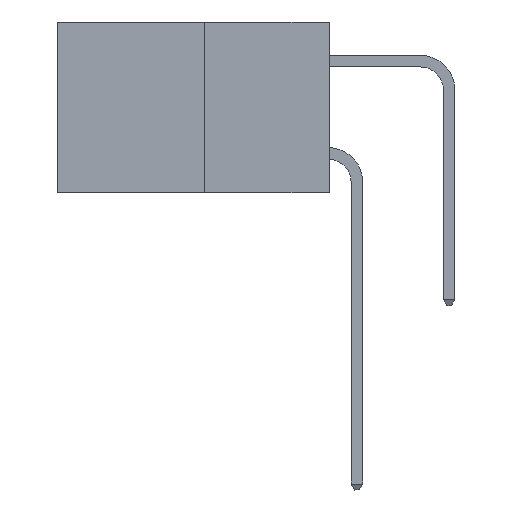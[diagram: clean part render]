
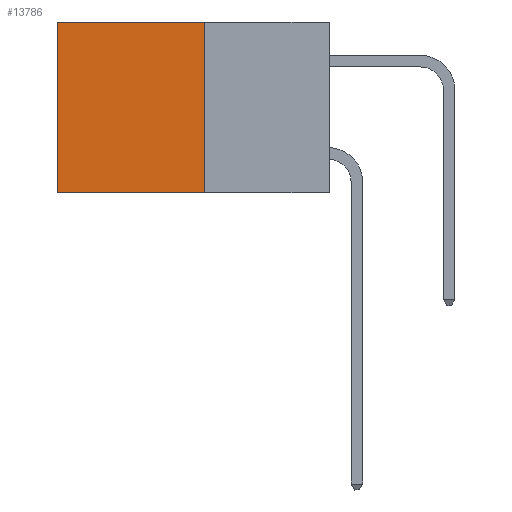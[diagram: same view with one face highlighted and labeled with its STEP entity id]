
A CAD part, left-side view. The second image highlights one B-rep face of the part: STEP entity #13786.
In plain terms, the highlighted planar face has unit normal (-1, 0, 0).
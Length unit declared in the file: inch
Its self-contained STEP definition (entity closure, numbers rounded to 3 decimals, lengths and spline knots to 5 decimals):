
#112 = DIRECTION ( 'NONE',  ( 0., 0., -1. ) ) ;
#153 = LINE ( 'NONE', #975, #4614 ) ;
#975 = CARTESIAN_POINT ( 'NONE',  ( 0.277, 0.27, -0.37 ) ) ;
#1062 = VERTEX_POINT ( 'NONE', #6786 ) ;
#1431 = CARTESIAN_POINT ( 'NONE',  ( 0.277, 0.59, -0.37 ) ) ;
#2430 = VECTOR ( 'NONE', #12693, 39.37008 ) ;
#3535 = CARTESIAN_POINT ( 'NONE',  ( 0.277, 0.27, -0.37 ) ) ;
#3615 = ORIENTED_EDGE ( 'NONE', *, *, #19193, .T. ) ;
#4493 = AXIS2_PLACEMENT_3D ( 'NONE', #22102, #11427, #112 ) ;
#4614 = VECTOR ( 'NONE', #19745, 39.37008 ) ;
#6786 = CARTESIAN_POINT ( 'NONE',  ( 0.277, 0.27, 0. ) ) ;
#7152 = CARTESIAN_POINT ( 'NONE',  ( 0.277, 0.59, -0.37 ) ) ;
#7329 = DIRECTION ( 'NONE',  ( 0., 0., -1. ) ) ;
#7361 = LINE ( 'NONE', #15673, #16532 ) ;
#7811 = VERTEX_POINT ( 'NONE', #7152 ) ;
#9044 = EDGE_CURVE ( 'NONE', #22969, #7811, #153, .T. ) ;
#9548 = PLANE ( 'NONE',  #4493 ) ;
#9680 = LINE ( 'NONE', #3535, #18723 ) ;
#11427 = DIRECTION ( 'NONE',  ( 1., 0., 0. ) ) ;
#12693 = DIRECTION ( 'NONE',  ( 0., 0., -1. ) ) ;
#13409 = ORIENTED_EDGE ( 'NONE', *, *, #17498, .T. ) ;
#13786 = ADVANCED_FACE ( 'NONE', ( #15715 ), #9548, .F. ) ;
#13839 = ORIENTED_EDGE ( 'NONE', *, *, #20639, .F. ) ;
#14053 = CARTESIAN_POINT ( 'NONE',  ( 0.277, 0.27, -0.37 ) ) ;
#14807 = EDGE_LOOP ( 'NONE', ( #13409, #18150, #13839, #3615 ) ) ;
#15673 = CARTESIAN_POINT ( 'NONE',  ( 0.277, 0.27, 0. ) ) ;
#15715 = FACE_OUTER_BOUND ( 'NONE', #14807, .T. ) ;
#16532 = VECTOR ( 'NONE', #17474, 39.37008 ) ;
#17474 = DIRECTION ( 'NONE',  ( 0., 1., 0. ) ) ;
#17498 = EDGE_CURVE ( 'NONE', #21939, #7811, #21880, .T. ) ;
#18150 = ORIENTED_EDGE ( 'NONE', *, *, #9044, .F. ) ;
#18723 = VECTOR ( 'NONE', #7329, 39.37008 ) ;
#19193 = EDGE_CURVE ( 'NONE', #1062, #21939, #7361, .T. ) ;
#19745 = DIRECTION ( 'NONE',  ( 0., 1., 0. ) ) ;
#19897 = CARTESIAN_POINT ( 'NONE',  ( 0.277, 0.59, 0. ) ) ;
#20639 = EDGE_CURVE ( 'NONE', #1062, #22969, #9680, .T. ) ;
#21880 = LINE ( 'NONE', #1431, #2430 ) ;
#21939 = VERTEX_POINT ( 'NONE', #19897 ) ;
#22102 = CARTESIAN_POINT ( 'NONE',  ( 0.277, 0.27, -0.37 ) ) ;
#22969 = VERTEX_POINT ( 'NONE', #14053 ) ;
